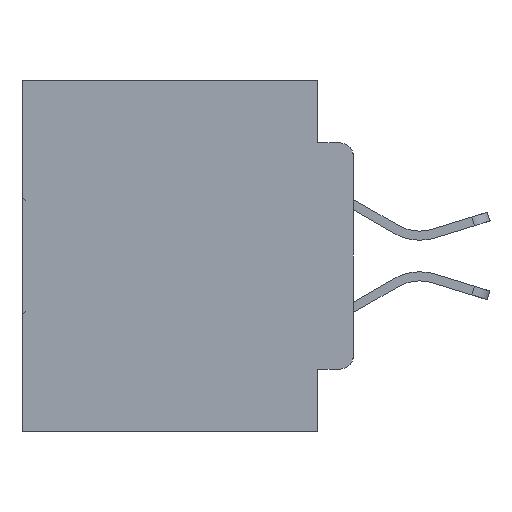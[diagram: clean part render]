
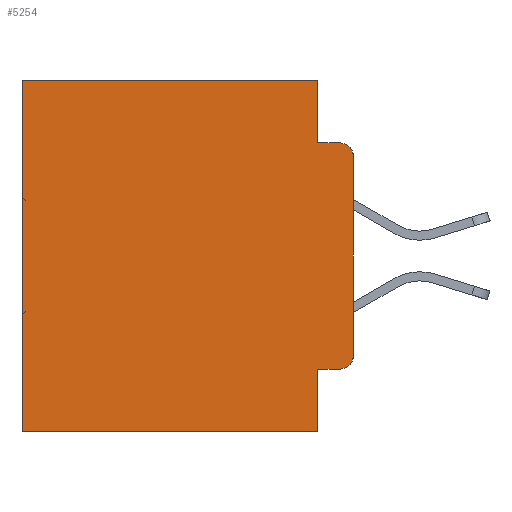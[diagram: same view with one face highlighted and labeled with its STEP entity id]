
A CAD part, left-side view. The second image highlights one B-rep face of the part: STEP entity #5254.
In plain terms, the highlighted planar face has unit normal (-1, 0, 0).
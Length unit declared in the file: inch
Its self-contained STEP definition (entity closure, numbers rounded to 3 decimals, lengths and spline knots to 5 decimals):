
#37 = CARTESIAN_POINT ( 'NONE',  ( 0.298, 0.051, -0.0885 ) ) ;
#62 = LINE ( 'NONE', #32944, #27821 ) ;
#838 = DIRECTION ( 'NONE',  ( 0., 0., -1. ) ) ;
#1249 = CARTESIAN_POINT ( 'NONE',  ( 0.298, 0., -0.3915 ) ) ;
#2042 = EDGE_LOOP ( 'NONE', ( #14455, #13036, #3921, #17837, #30359, #21383, #26006, #7135, #18046, #29006 ) ) ;
#2183 = CARTESIAN_POINT ( 'NONE',  ( 0.298, 0.02, -0.4115 ) ) ;
#2196 = VERTEX_POINT ( 'NONE', #34060 ) ;
#2220 = DIRECTION ( 'NONE',  ( 0., 0., -1. ) ) ;
#3442 = CARTESIAN_POINT ( 'NONE',  ( 0.298, 0.02, -0.3915 ) ) ;
#3682 = VERTEX_POINT ( 'NONE', #11684 ) ;
#3764 = DIRECTION ( 'NONE',  ( 0., 0., -1. ) ) ;
#3921 = ORIENTED_EDGE ( 'NONE', *, *, #14804, .F. ) ;
#4457 = VECTOR ( 'NONE', #7363, 39.37008 ) ;
#4858 = EDGE_CURVE ( 'NONE', #2196, #12421, #29743, .T. ) ;
#5094 = CARTESIAN_POINT ( 'NONE',  ( 0.298, 0.473, 0. ) ) ;
#5254 = ADVANCED_FACE ( 'NONE', ( #34822 ), #27642, .F. ) ;
#5457 = VERTEX_POINT ( 'NONE', #11954 ) ;
#6193 = CIRCLE ( 'NONE', #22633, 0.02 ) ;
#7135 = ORIENTED_EDGE ( 'NONE', *, *, #11904, .F. ) ;
#7363 = DIRECTION ( 'NONE',  ( 0., 1., 0. ) ) ;
#7557 = CARTESIAN_POINT ( 'NONE',  ( 0.298, 0.051, 0. ) ) ;
#7925 = VECTOR ( 'NONE', #28461, 39.37008 ) ;
#8878 = DIRECTION ( 'NONE',  ( -1., 0., 0. ) ) ;
#9676 = EDGE_CURVE ( 'NONE', #2196, #29878, #27984, .T. ) ;
#10951 = VERTEX_POINT ( 'NONE', #28554 ) ;
#11136 = DIRECTION ( 'NONE',  ( 0., -1., 0. ) ) ;
#11419 = CARTESIAN_POINT ( 'NONE',  ( 0.298, 0.473, -0.5 ) ) ;
#11684 = CARTESIAN_POINT ( 'NONE',  ( 0.298, 0., -0.1085 ) ) ;
#11904 = EDGE_CURVE ( 'NONE', #10951, #13941, #19460, .T. ) ;
#11954 = CARTESIAN_POINT ( 'NONE',  ( 0.298, 0.02, -0.0885 ) ) ;
#12264 = CARTESIAN_POINT ( 'NONE',  ( 0.298, 0.051, -0.5 ) ) ;
#12421 = VERTEX_POINT ( 'NONE', #5094 ) ;
#12728 = VECTOR ( 'NONE', #16655, 39.37008 ) ;
#12957 = VECTOR ( 'NONE', #11136, 39.37008 ) ;
#13036 = ORIENTED_EDGE ( 'NONE', *, *, #18140, .T. ) ;
#13941 = VERTEX_POINT ( 'NONE', #12264 ) ;
#14455 = ORIENTED_EDGE ( 'NONE', *, *, #30835, .F. ) ;
#14582 = AXIS2_PLACEMENT_3D ( 'NONE', #21983, #26352, #2220 ) ;
#14804 = EDGE_CURVE ( 'NONE', #29878, #5457, #31858, .T. ) ;
#15317 = EDGE_CURVE ( 'NONE', #13941, #17968, #32643, .T. ) ;
#15724 = LINE ( 'NONE', #16993, #28727 ) ;
#15795 = DIRECTION ( 'NONE',  ( 0., 0., -1. ) ) ;
#16655 = DIRECTION ( 'NONE',  ( 0., 0., -1. ) ) ;
#16842 = DIRECTION ( 'NONE',  ( 0., -1., 0. ) ) ;
#16929 = VECTOR ( 'NONE', #15795, 39.37008 ) ;
#16993 = CARTESIAN_POINT ( 'NONE',  ( 0.298, 0.473, 0. ) ) ;
#17837 = ORIENTED_EDGE ( 'NONE', *, *, #9676, .F. ) ;
#17968 = VERTEX_POINT ( 'NONE', #11419 ) ;
#18046 = ORIENTED_EDGE ( 'NONE', *, *, #31573, .T. ) ;
#18140 = EDGE_CURVE ( 'NONE', #3682, #5457, #28994, .T. ) ;
#19460 = LINE ( 'NONE', #7557, #16929 ) ;
#19917 = DIRECTION ( 'NONE',  ( 1., 0., 0. ) ) ;
#20439 = VERTEX_POINT ( 'NONE', #1249 ) ;
#21372 = AXIS2_PLACEMENT_3D ( 'NONE', #33329, #19917, #3764 ) ;
#21383 = ORIENTED_EDGE ( 'NONE', *, *, #29728, .T. ) ;
#21930 = LINE ( 'NONE', #26967, #12728 ) ;
#21983 = CARTESIAN_POINT ( 'NONE',  ( 0.298, 0.02, -0.1085 ) ) ;
#22633 = AXIS2_PLACEMENT_3D ( 'NONE', #3442, #8878, #28364 ) ;
#22939 = CARTESIAN_POINT ( 'NONE',  ( 0.298, 0., 0. ) ) ;
#23378 = VECTOR ( 'NONE', #27956, 39.37008 ) ;
#26006 = ORIENTED_EDGE ( 'NONE', *, *, #15317, .F. ) ;
#26352 = DIRECTION ( 'NONE',  ( -1., 0., 0. ) ) ;
#26967 = CARTESIAN_POINT ( 'NONE',  ( 0.298, 0., 0. ) ) ;
#27642 = PLANE ( 'NONE',  #21372 ) ;
#27821 = VECTOR ( 'NONE', #16842, 39.37008 ) ;
#27956 = DIRECTION ( 'NONE',  ( 0., 0., -1. ) ) ;
#27984 = LINE ( 'NONE', #30905, #23378 ) ;
#28364 = DIRECTION ( 'NONE',  ( 0., 0., -1. ) ) ;
#28461 = DIRECTION ( 'NONE',  ( 0., 1., 0. ) ) ;
#28554 = CARTESIAN_POINT ( 'NONE',  ( 0.298, 0.051, -0.4115 ) ) ;
#28727 = VECTOR ( 'NONE', #838, 39.37008 ) ;
#28994 = CIRCLE ( 'NONE', #14582, 0.02 ) ;
#29006 = ORIENTED_EDGE ( 'NONE', *, *, #34001, .T. ) ;
#29728 = EDGE_CURVE ( 'NONE', #12421, #17968, #15724, .T. ) ;
#29743 = LINE ( 'NONE', #22939, #7925 ) ;
#29878 = VERTEX_POINT ( 'NONE', #33195 ) ;
#30359 = ORIENTED_EDGE ( 'NONE', *, *, #4858, .T. ) ;
#30835 = EDGE_CURVE ( 'NONE', #3682, #20439, #21930, .T. ) ;
#30905 = CARTESIAN_POINT ( 'NONE',  ( 0.298, 0.051, 0. ) ) ;
#31573 = EDGE_CURVE ( 'NONE', #10951, #33515, #62, .T. ) ;
#31858 = LINE ( 'NONE', #37, #12957 ) ;
#32643 = LINE ( 'NONE', #34176, #4457 ) ;
#32944 = CARTESIAN_POINT ( 'NONE',  ( 0.298, 0.051, -0.4115 ) ) ;
#33195 = CARTESIAN_POINT ( 'NONE',  ( 0.298, 0.051, -0.0885 ) ) ;
#33329 = CARTESIAN_POINT ( 'NONE',  ( 0.298, 0., 0. ) ) ;
#33515 = VERTEX_POINT ( 'NONE', #2183 ) ;
#34001 = EDGE_CURVE ( 'NONE', #33515, #20439, #6193, .T. ) ;
#34060 = CARTESIAN_POINT ( 'NONE',  ( 0.298, 0.051, 0. ) ) ;
#34176 = CARTESIAN_POINT ( 'NONE',  ( 0.298, 0., -0.5 ) ) ;
#34822 = FACE_OUTER_BOUND ( 'NONE', #2042, .T. ) ;
